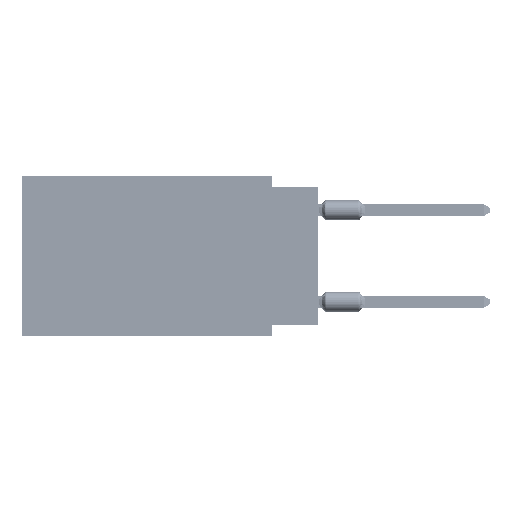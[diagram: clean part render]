
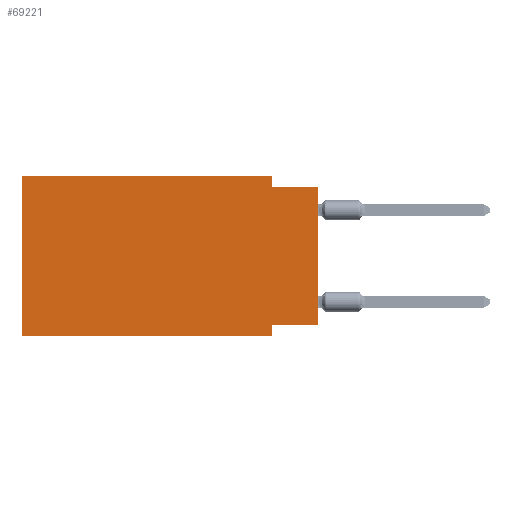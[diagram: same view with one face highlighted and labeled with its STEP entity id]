
A CAD part, left-side view. The second image highlights one B-rep face of the part: STEP entity #69221.
In plain terms, the highlighted planar face has unit normal (-1, 0, 0).
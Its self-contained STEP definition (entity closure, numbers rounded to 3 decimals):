
#149 = EDGE_CURVE ( 'NONE', #61138, #61583, #22623, .T. ) ;
#1985 = VERTEX_POINT ( 'NONE', #52939 ) ;
#2214 = DIRECTION ( 'NONE',  ( 0., -1., 0. ) ) ;
#2749 = ORIENTED_EDGE ( 'NONE', *, *, #46657, .T. ) ;
#3367 = CARTESIAN_POINT ( 'NONE',  ( 0., 2.54, -8.255 ) ) ;
#4133 = CARTESIAN_POINT ( 'NONE',  ( 0., 16.383, 0. ) ) ;
#4157 = DIRECTION ( 'NONE',  ( 0., 0., 1. ) ) ;
#4409 = LINE ( 'NONE', #64514, #28743 ) ;
#6668 = CARTESIAN_POINT ( 'NONE',  ( 0., 2.54, -0.635 ) ) ;
#6842 = VERTEX_POINT ( 'NONE', #3367 ) ;
#7114 = VECTOR ( 'NONE', #40989, 1000. ) ;
#7341 = CARTESIAN_POINT ( 'NONE',  ( 0., 0., -0.635 ) ) ;
#8432 = DIRECTION ( 'NONE',  ( 1., 0., 0. ) ) ;
#8783 = EDGE_CURVE ( 'NONE', #61583, #67972, #47078, .T. ) ;
#9010 = CARTESIAN_POINT ( 'NONE',  ( 0., 2.54, -8.89 ) ) ;
#10122 = DIRECTION ( 'NONE',  ( 0., 1., 0. ) ) ;
#12188 = EDGE_LOOP ( 'NONE', ( #2749, #22146, #15586, #54109, #38687, #18254, #35239, #42803 ) ) ;
#13093 = VERTEX_POINT ( 'NONE', #53790 ) ;
#15323 = CARTESIAN_POINT ( 'NONE',  ( 0., 16.383, 0. ) ) ;
#15586 = ORIENTED_EDGE ( 'NONE', *, *, #8783, .F. ) ;
#18254 = ORIENTED_EDGE ( 'NONE', *, *, #68821, .T. ) ;
#19988 = LINE ( 'NONE', #46823, #33205 ) ;
#20678 = LINE ( 'NONE', #62911, #57625 ) ;
#22146 = ORIENTED_EDGE ( 'NONE', *, *, #48854, .F. ) ;
#22623 = LINE ( 'NONE', #56608, #64614 ) ;
#23826 = EDGE_CURVE ( 'NONE', #1985, #6842, #4409, .T. ) ;
#28743 = VECTOR ( 'NONE', #10122, 1000. ) ;
#30242 = DIRECTION ( 'NONE',  ( 0., 0., -1. ) ) ;
#30990 = LINE ( 'NONE', #42436, #48028 ) ;
#33205 = VECTOR ( 'NONE', #63642, 1000. ) ;
#33271 = CARTESIAN_POINT ( 'NONE',  ( 0., 16.383, 0. ) ) ;
#35239 = ORIENTED_EDGE ( 'NONE', *, *, #46664, .F. ) ;
#38687 = ORIENTED_EDGE ( 'NONE', *, *, #45099, .F. ) ;
#40989 = DIRECTION ( 'NONE',  ( 0., 0., -1. ) ) ;
#42436 = CARTESIAN_POINT ( 'NONE',  ( 0., 2.54, -8.89 ) ) ;
#42803 = ORIENTED_EDGE ( 'NONE', *, *, #23826, .F. ) ;
#45099 = EDGE_CURVE ( 'NONE', #13093, #61138, #47177, .T. ) ;
#46372 = CARTESIAN_POINT ( 'NONE',  ( 0., 2.54, 0. ) ) ;
#46657 = EDGE_CURVE ( 'NONE', #1985, #64423, #58890, .T. ) ;
#46664 = EDGE_CURVE ( 'NONE', #6842, #55869, #30990, .T. ) ;
#46707 = PLANE ( 'NONE',  #55234 ) ;
#46823 = CARTESIAN_POINT ( 'NONE',  ( 0., 0., -0.635 ) ) ;
#47078 = LINE ( 'NONE', #47783, #7114 ) ;
#47177 = LINE ( 'NONE', #15323, #64997 ) ;
#47783 = CARTESIAN_POINT ( 'NONE',  ( 0., 2.54, 0. ) ) ;
#48028 = VECTOR ( 'NONE', #52828, 1000. ) ;
#48854 = EDGE_CURVE ( 'NONE', #67972, #64423, #19988, .T. ) ;
#52828 = DIRECTION ( 'NONE',  ( 0., 0., -1. ) ) ;
#52939 = CARTESIAN_POINT ( 'NONE',  ( 0., 0., -8.255 ) ) ;
#53790 = CARTESIAN_POINT ( 'NONE',  ( 0., 16.383, -8.89 ) ) ;
#54109 = ORIENTED_EDGE ( 'NONE', *, *, #149, .F. ) ;
#55234 = AXIS2_PLACEMENT_3D ( 'NONE', #4133, #8432, #30242 ) ;
#55869 = VERTEX_POINT ( 'NONE', #9010 ) ;
#56608 = CARTESIAN_POINT ( 'NONE',  ( 0., 16.383, 0. ) ) ;
#57538 = DIRECTION ( 'NONE',  ( 0., -1., 0. ) ) ;
#57625 = VECTOR ( 'NONE', #57538, 1000. ) ;
#58300 = VECTOR ( 'NONE', #4157, 1000. ) ;
#58890 = LINE ( 'NONE', #63204, #58300 ) ;
#58965 = DIRECTION ( 'NONE',  ( 0., 0., 1. ) ) ;
#61138 = VERTEX_POINT ( 'NONE', #33271 ) ;
#61583 = VERTEX_POINT ( 'NONE', #46372 ) ;
#62911 = CARTESIAN_POINT ( 'NONE',  ( 0., 16.383, -8.89 ) ) ;
#63204 = CARTESIAN_POINT ( 'NONE',  ( 0., 0., 0. ) ) ;
#63642 = DIRECTION ( 'NONE',  ( 0., -1., 0. ) ) ;
#64423 = VERTEX_POINT ( 'NONE', #7341 ) ;
#64514 = CARTESIAN_POINT ( 'NONE',  ( 0., 0., -8.255 ) ) ;
#64614 = VECTOR ( 'NONE', #2214, 1000. ) ;
#64997 = VECTOR ( 'NONE', #58965, 1000. ) ;
#67972 = VERTEX_POINT ( 'NONE', #6668 ) ;
#68821 = EDGE_CURVE ( 'NONE', #13093, #55869, #20678, .T. ) ;
#69221 = ADVANCED_FACE ( 'NONE', ( #69594 ), #46707, .F. ) ;
#69594 = FACE_OUTER_BOUND ( 'NONE', #12188, .T. ) ;
